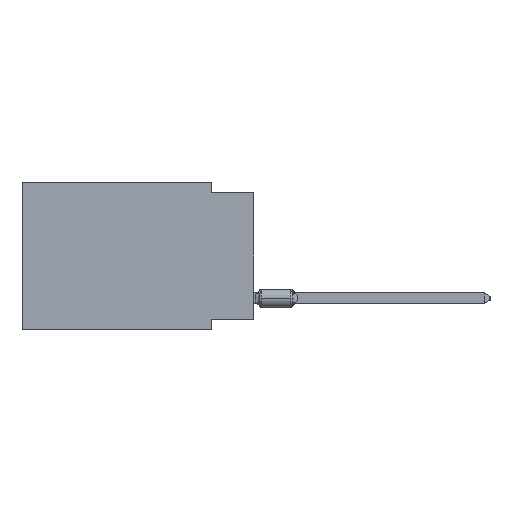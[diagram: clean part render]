
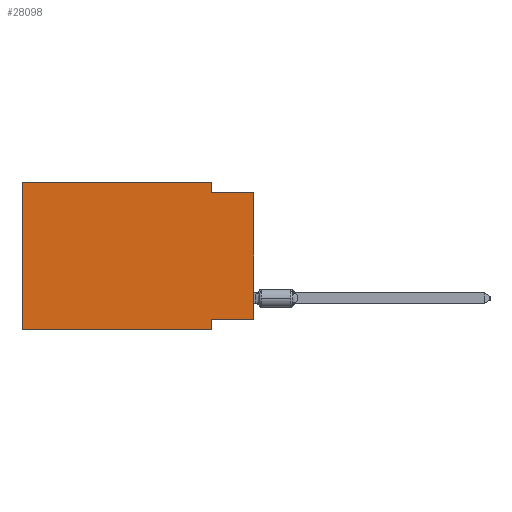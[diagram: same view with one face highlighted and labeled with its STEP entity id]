
A CAD part, left-side view. The second image highlights one B-rep face of the part: STEP entity #28098.
In plain terms, the highlighted planar face has unit normal (-1, 0, 0).
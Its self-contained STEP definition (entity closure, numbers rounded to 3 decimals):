
#142 = EDGE_CURVE ( 'NONE', #33985, #4578, #14899, .T. ) ;
#249 = EDGE_CURVE ( 'NONE', #4578, #25905, #47006, .T. ) ;
#702 = ORIENTED_EDGE ( 'NONE', *, *, #142, .F. ) ;
#4578 = VERTEX_POINT ( 'NONE', #21110 ) ;
#5026 = EDGE_LOOP ( 'NONE', ( #9502, #10284, #45714, #27197, #702, #55416, #43624, #50870 ) ) ;
#5033 = VECTOR ( 'NONE', #52826, 1000. ) ;
#5515 = DIRECTION ( 'NONE',  ( 0., -1., 0. ) ) ;
#5779 = DIRECTION ( 'NONE',  ( 0., 1., 0. ) ) ;
#5782 = CARTESIAN_POINT ( 'NONE',  ( 0., 13.97, 0. ) ) ;
#6795 = DIRECTION ( 'NONE',  ( 0., -1., 0. ) ) ;
#7986 = VERTEX_POINT ( 'NONE', #40632 ) ;
#8004 = CARTESIAN_POINT ( 'NONE',  ( 0., 2.54, 0. ) ) ;
#9502 = ORIENTED_EDGE ( 'NONE', *, *, #39644, .T. ) ;
#9555 = CARTESIAN_POINT ( 'NONE',  ( 0., 0., -8.255 ) ) ;
#10284 = ORIENTED_EDGE ( 'NONE', *, *, #31248, .F. ) ;
#10569 = DIRECTION ( 'NONE',  ( 0., 0., 1. ) ) ;
#12695 = EDGE_CURVE ( 'NONE', #25905, #7986, #16982, .T. ) ;
#12961 = CARTESIAN_POINT ( 'NONE',  ( 0., 2.54, -8.255 ) ) ;
#12966 = VECTOR ( 'NONE', #29331, 1000. ) ;
#13463 = CARTESIAN_POINT ( 'NONE',  ( 0., 2.54, -8.89 ) ) ;
#14899 = LINE ( 'NONE', #54255, #47408 ) ;
#15172 = CARTESIAN_POINT ( 'NONE',  ( 0., 13.97, -8.89 ) ) ;
#15790 = CARTESIAN_POINT ( 'NONE',  ( 0., 0., -0.635 ) ) ;
#16034 = CARTESIAN_POINT ( 'NONE',  ( 0., 13.97, 0. ) ) ;
#16133 = EDGE_CURVE ( 'NONE', #49281, #46153, #26913, .T. ) ;
#16982 = LINE ( 'NONE', #8004, #40003 ) ;
#17964 = LINE ( 'NONE', #44297, #40834 ) ;
#20724 = EDGE_CURVE ( 'NONE', #33985, #39664, #17964, .T. ) ;
#21110 = CARTESIAN_POINT ( 'NONE',  ( 0., 13.97, 0. ) ) ;
#21301 = LINE ( 'NONE', #30841, #5033 ) ;
#21726 = CARTESIAN_POINT ( 'NONE',  ( 0., 2.54, -8.89 ) ) ;
#22751 = CARTESIAN_POINT ( 'NONE',  ( 0., 0., -0.635 ) ) ;
#23425 = DIRECTION ( 'NONE',  ( 1., 0., 0. ) ) ;
#25905 = VERTEX_POINT ( 'NONE', #32903 ) ;
#26913 = LINE ( 'NONE', #9555, #40211 ) ;
#27197 = ORIENTED_EDGE ( 'NONE', *, *, #249, .F. ) ;
#28098 = ADVANCED_FACE ( 'NONE', ( #36453 ), #45415, .F. ) ;
#28833 = DIRECTION ( 'NONE',  ( 0., -1., 0. ) ) ;
#29331 = DIRECTION ( 'NONE',  ( 0., 0., -1. ) ) ;
#29522 = AXIS2_PLACEMENT_3D ( 'NONE', #5782, #23425, #44848 ) ;
#30312 = EDGE_CURVE ( 'NONE', #46153, #39664, #31278, .T. ) ;
#30841 = CARTESIAN_POINT ( 'NONE',  ( 0., 0., 0. ) ) ;
#31248 = EDGE_CURVE ( 'NONE', #7986, #45246, #33729, .T. ) ;
#31278 = LINE ( 'NONE', #21726, #12966 ) ;
#32903 = CARTESIAN_POINT ( 'NONE',  ( 0., 2.54, 0. ) ) ;
#33729 = LINE ( 'NONE', #15790, #39817 ) ;
#33985 = VERTEX_POINT ( 'NONE', #15172 ) ;
#34917 = DIRECTION ( 'NONE',  ( 0., 0., -1. ) ) ;
#36453 = FACE_OUTER_BOUND ( 'NONE', #5026, .T. ) ;
#39644 = EDGE_CURVE ( 'NONE', #49281, #45246, #21301, .T. ) ;
#39664 = VERTEX_POINT ( 'NONE', #13463 ) ;
#39817 = VECTOR ( 'NONE', #28833, 1000. ) ;
#40003 = VECTOR ( 'NONE', #34917, 1000. ) ;
#40211 = VECTOR ( 'NONE', #5779, 1000. ) ;
#40632 = CARTESIAN_POINT ( 'NONE',  ( 0., 2.54, -0.635 ) ) ;
#40834 = VECTOR ( 'NONE', #5515, 1000. ) ;
#43624 = ORIENTED_EDGE ( 'NONE', *, *, #30312, .F. ) ;
#44297 = CARTESIAN_POINT ( 'NONE',  ( 0., 13.97, -8.89 ) ) ;
#44848 = DIRECTION ( 'NONE',  ( 0., 0., -1. ) ) ;
#45246 = VERTEX_POINT ( 'NONE', #22751 ) ;
#45415 = PLANE ( 'NONE',  #29522 ) ;
#45714 = ORIENTED_EDGE ( 'NONE', *, *, #12695, .F. ) ;
#46153 = VERTEX_POINT ( 'NONE', #12961 ) ;
#46485 = CARTESIAN_POINT ( 'NONE',  ( 0., 0., -8.255 ) ) ;
#47006 = LINE ( 'NONE', #16034, #55709 ) ;
#47408 = VECTOR ( 'NONE', #10569, 1000. ) ;
#49281 = VERTEX_POINT ( 'NONE', #46485 ) ;
#50870 = ORIENTED_EDGE ( 'NONE', *, *, #16133, .F. ) ;
#52826 = DIRECTION ( 'NONE',  ( 0., 0., 1. ) ) ;
#54255 = CARTESIAN_POINT ( 'NONE',  ( 0., 13.97, 0. ) ) ;
#55416 = ORIENTED_EDGE ( 'NONE', *, *, #20724, .T. ) ;
#55709 = VECTOR ( 'NONE', #6795, 1000. ) ;
